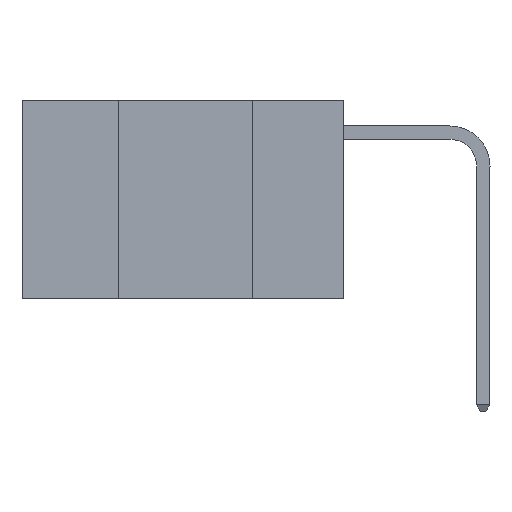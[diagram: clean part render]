
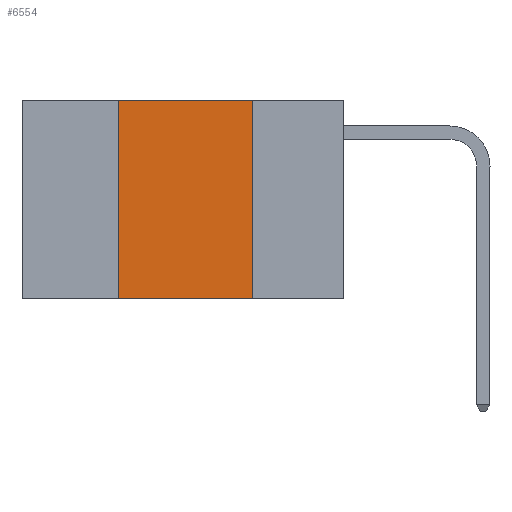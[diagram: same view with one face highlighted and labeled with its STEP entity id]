
A CAD part, left-side view. The second image highlights one B-rep face of the part: STEP entity #6554.
In plain terms, the highlighted planar face has unit normal (-1, 0, 0).
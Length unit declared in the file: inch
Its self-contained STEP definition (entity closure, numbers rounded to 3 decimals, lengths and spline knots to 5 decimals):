
#17 = CARTESIAN_POINT ( 'NONE',  ( 0., 0.42, 0. ) ) ;
#23 = CARTESIAN_POINT ( 'NONE',  ( 0., 0.17, -0.37 ) ) ;
#1217 = EDGE_CURVE ( 'NONE', #6727, #11542, #5186, .T. ) ;
#1620 = CARTESIAN_POINT ( 'NONE',  ( 0., 0.42, -0.37 ) ) ;
#1764 = EDGE_LOOP ( 'NONE', ( #5244, #10922, #2721, #5578 ) ) ;
#2233 = DIRECTION ( 'NONE',  ( 0., 0., -1. ) ) ;
#2409 = CARTESIAN_POINT ( 'NONE',  ( 0., 0.6, 0. ) ) ;
#2501 = EDGE_CURVE ( 'NONE', #13052, #11550, #5486, .T. ) ;
#2527 = CARTESIAN_POINT ( 'NONE',  ( 0., 0.6, -0.37 ) ) ;
#2721 = ORIENTED_EDGE ( 'NONE', *, *, #10840, .F. ) ;
#2957 = EDGE_CURVE ( 'NONE', #11550, #11542, #2962, .T. ) ;
#2962 = LINE ( 'NONE', #3255, #7971 ) ;
#3255 = CARTESIAN_POINT ( 'NONE',  ( 0., 0.17, 0. ) ) ;
#3346 = CARTESIAN_POINT ( 'NONE',  ( 0., 0.17, 0. ) ) ;
#3495 = DIRECTION ( 'NONE',  ( 1., 0., 0. ) ) ;
#4026 = CARTESIAN_POINT ( 'NONE',  ( 0., 0.42, 0. ) ) ;
#4789 = CARTESIAN_POINT ( 'NONE',  ( 0., 0.6, 0. ) ) ;
#5186 = LINE ( 'NONE', #2527, #7694 ) ;
#5244 = ORIENTED_EDGE ( 'NONE', *, *, #2957, .F. ) ;
#5486 = LINE ( 'NONE', #4789, #13630 ) ;
#5578 = ORIENTED_EDGE ( 'NONE', *, *, #1217, .T. ) ;
#5856 = DIRECTION ( 'NONE',  ( 0., -1., 0. ) ) ;
#6554 = ADVANCED_FACE ( 'NONE', ( #7718 ), #8806, .F. ) ;
#6727 = VERTEX_POINT ( 'NONE', #1620 ) ;
#7569 = DIRECTION ( 'NONE',  ( 0., 0., 1. ) ) ;
#7694 = VECTOR ( 'NONE', #9983, 39.37008 ) ;
#7718 = FACE_OUTER_BOUND ( 'NONE', #1764, .T. ) ;
#7971 = VECTOR ( 'NONE', #2233, 39.37008 ) ;
#8806 = PLANE ( 'NONE',  #12127 ) ;
#9983 = DIRECTION ( 'NONE',  ( 0., -1., 0. ) ) ;
#10840 = EDGE_CURVE ( 'NONE', #6727, #13052, #12732, .T. ) ;
#10922 = ORIENTED_EDGE ( 'NONE', *, *, #2501, .F. ) ;
#10947 = DIRECTION ( 'NONE',  ( 0., 0., -1. ) ) ;
#11542 = VERTEX_POINT ( 'NONE', #23 ) ;
#11550 = VERTEX_POINT ( 'NONE', #3346 ) ;
#12127 = AXIS2_PLACEMENT_3D ( 'NONE', #2409, #3495, #10947 ) ;
#12396 = VECTOR ( 'NONE', #7569, 39.37008 ) ;
#12732 = LINE ( 'NONE', #17, #12396 ) ;
#13052 = VERTEX_POINT ( 'NONE', #4026 ) ;
#13630 = VECTOR ( 'NONE', #5856, 39.37008 ) ;
